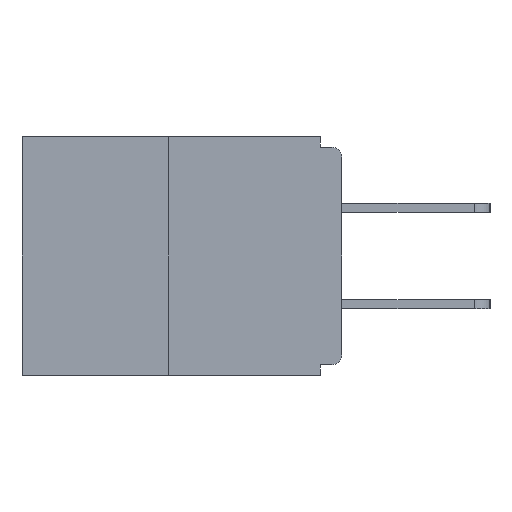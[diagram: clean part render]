
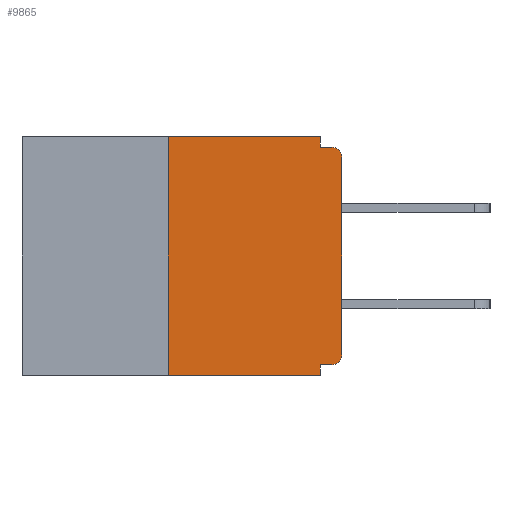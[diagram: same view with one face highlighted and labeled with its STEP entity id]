
A CAD part, left-side view. The second image highlights one B-rep face of the part: STEP entity #9865.
In plain terms, the highlighted planar face has unit normal (-1, 0, 0).
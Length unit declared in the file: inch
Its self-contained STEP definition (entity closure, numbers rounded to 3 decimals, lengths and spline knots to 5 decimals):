
#80 = LINE ( 'NONE', #8680, #6039 ) ;
#93 = DIRECTION ( 'NONE',  ( 1., 0., 0. ) ) ;
#171 = EDGE_CURVE ( 'NONE', #6307, #4086, #8554, .T. ) ;
#205 = CARTESIAN_POINT ( 'NONE',  ( 0., 0.031, -0.328 ) ) ;
#256 = VERTEX_POINT ( 'NONE', #938 ) ;
#393 = CARTESIAN_POINT ( 'NONE',  ( 0., 0.015, -0.015 ) ) ;
#521 = DIRECTION ( 'NONE',  ( 0., -1., 0. ) ) ;
#561 = VERTEX_POINT ( 'NONE', #637 ) ;
#637 = CARTESIAN_POINT ( 'NONE',  ( 0., 0.031, -0.015 ) ) ;
#755 = CARTESIAN_POINT ( 'NONE',  ( 0., 0.25, 0. ) ) ;
#938 = CARTESIAN_POINT ( 'NONE',  ( 0., 0., -0.313 ) ) ;
#1187 = EDGE_CURVE ( 'NONE', #561, #4008, #1650, .T. ) ;
#1219 = EDGE_CURVE ( 'NONE', #5579, #256, #6534, .T. ) ;
#1483 = DIRECTION ( 'NONE',  ( 0., 0., -1. ) ) ;
#1650 = LINE ( 'NONE', #8411, #4233 ) ;
#2197 = VERTEX_POINT ( 'NONE', #205 ) ;
#2252 = CARTESIAN_POINT ( 'NONE',  ( 0., 0.25, 0. ) ) ;
#2537 = CARTESIAN_POINT ( 'NONE',  ( 0., 0.031, 0. ) ) ;
#3429 = CARTESIAN_POINT ( 'NONE',  ( 0., 0.015, -0.313 ) ) ;
#3512 = LINE ( 'NONE', #12268, #11668 ) ;
#3751 = VECTOR ( 'NONE', #4068, 39.37008 ) ;
#4008 = VERTEX_POINT ( 'NONE', #393 ) ;
#4068 = DIRECTION ( 'NONE',  ( 0., 0., 1. ) ) ;
#4086 = VERTEX_POINT ( 'NONE', #2537 ) ;
#4202 = ORIENTED_EDGE ( 'NONE', *, *, #5926, .F. ) ;
#4233 = VECTOR ( 'NONE', #521, 39.37008 ) ;
#4333 = CARTESIAN_POINT ( 'NONE',  ( 0., 0.031, 0. ) ) ;
#4371 = AXIS2_PLACEMENT_3D ( 'NONE', #11123, #12133, #6259 ) ;
#5271 = FACE_OUTER_BOUND ( 'NONE', #10379, .T. ) ;
#5474 = DIRECTION ( 'NONE',  ( 0., 0., -1. ) ) ;
#5579 = VERTEX_POINT ( 'NONE', #8364 ) ;
#5926 = EDGE_CURVE ( 'NONE', #2197, #12095, #3512, .T. ) ;
#6029 = CARTESIAN_POINT ( 'NONE',  ( 0., 0.46, 0. ) ) ;
#6039 = VECTOR ( 'NONE', #9717, 39.37008 ) ;
#6090 = VERTEX_POINT ( 'NONE', #10890 ) ;
#6117 = AXIS2_PLACEMENT_3D ( 'NONE', #3429, #12184, #1483 ) ;
#6259 = DIRECTION ( 'NONE',  ( 0., 0., -1. ) ) ;
#6307 = VERTEX_POINT ( 'NONE', #755 ) ;
#6522 = LINE ( 'NONE', #2252, #3751 ) ;
#6534 = CIRCLE ( 'NONE', #6117, 0.015 ) ;
#6861 = AXIS2_PLACEMENT_3D ( 'NONE', #6029, #93, #10900 ) ;
#6955 = DIRECTION ( 'NONE',  ( 0., -1., 0. ) ) ;
#7190 = CARTESIAN_POINT ( 'NONE',  ( 0., 0., -0.328 ) ) ;
#7238 = CARTESIAN_POINT ( 'NONE',  ( 0., 0.25, -0.343 ) ) ;
#7279 = LINE ( 'NONE', #10842, #11589 ) ;
#7344 = EDGE_CURVE ( 'NONE', #4086, #561, #11327, .T. ) ;
#7654 = ORIENTED_EDGE ( 'NONE', *, *, #7344, .F. ) ;
#7789 = CARTESIAN_POINT ( 'NONE',  ( 0., 0.46, 0. ) ) ;
#7793 = VECTOR ( 'NONE', #12306, 39.37008 ) ;
#7835 = EDGE_CURVE ( 'NONE', #6090, #4008, #9789, .T. ) ;
#7993 = DIRECTION ( 'NONE',  ( 0., 0., 1. ) ) ;
#8178 = DIRECTION ( 'NONE',  ( 0., 1., 0. ) ) ;
#8364 = CARTESIAN_POINT ( 'NONE',  ( 0., 0.015, -0.328 ) ) ;
#8411 = CARTESIAN_POINT ( 'NONE',  ( 0., 0., -0.015 ) ) ;
#8523 = EDGE_CURVE ( 'NONE', #5579, #2197, #11895, .T. ) ;
#8554 = LINE ( 'NONE', #7789, #11791 ) ;
#8680 = CARTESIAN_POINT ( 'NONE',  ( 0., 0.46, -0.343 ) ) ;
#9605 = VECTOR ( 'NONE', #8178, 39.37008 ) ;
#9690 = EDGE_CURVE ( 'NONE', #10013, #12095, #80, .T. ) ;
#9717 = DIRECTION ( 'NONE',  ( 0., -1., 0. ) ) ;
#9789 = CIRCLE ( 'NONE', #4371, 0.015 ) ;
#9865 = ADVANCED_FACE ( 'NONE', ( #5271 ), #9926, .F. ) ;
#9926 = PLANE ( 'NONE',  #6861 ) ;
#10013 = VERTEX_POINT ( 'NONE', #7238 ) ;
#10192 = ORIENTED_EDGE ( 'NONE', *, *, #1219, .T. ) ;
#10379 = EDGE_LOOP ( 'NONE', ( #11484, #11418, #11967, #4202, #12081, #10192, #11290, #12413, #12439, #7654 ) ) ;
#10842 = CARTESIAN_POINT ( 'NONE',  ( 0., 0., 0. ) ) ;
#10890 = CARTESIAN_POINT ( 'NONE',  ( 0., 0., -0.03 ) ) ;
#10900 = DIRECTION ( 'NONE',  ( 0., 0., -1. ) ) ;
#11123 = CARTESIAN_POINT ( 'NONE',  ( 0., 0.015, -0.03 ) ) ;
#11228 = EDGE_CURVE ( 'NONE', #10013, #6307, #6522, .T. ) ;
#11290 = ORIENTED_EDGE ( 'NONE', *, *, #12100, .T. ) ;
#11327 = LINE ( 'NONE', #4333, #7793 ) ;
#11418 = ORIENTED_EDGE ( 'NONE', *, *, #11228, .F. ) ;
#11484 = ORIENTED_EDGE ( 'NONE', *, *, #171, .F. ) ;
#11589 = VECTOR ( 'NONE', #7993, 39.37008 ) ;
#11668 = VECTOR ( 'NONE', #5474, 39.37008 ) ;
#11791 = VECTOR ( 'NONE', #6955, 39.37008 ) ;
#11895 = LINE ( 'NONE', #7190, #9605 ) ;
#11937 = CARTESIAN_POINT ( 'NONE',  ( 0., 0.031, -0.343 ) ) ;
#11967 = ORIENTED_EDGE ( 'NONE', *, *, #9690, .T. ) ;
#12081 = ORIENTED_EDGE ( 'NONE', *, *, #8523, .F. ) ;
#12095 = VERTEX_POINT ( 'NONE', #11937 ) ;
#12100 = EDGE_CURVE ( 'NONE', #256, #6090, #7279, .T. ) ;
#12133 = DIRECTION ( 'NONE',  ( -1., 0., 0. ) ) ;
#12184 = DIRECTION ( 'NONE',  ( -1., 0., 0. ) ) ;
#12268 = CARTESIAN_POINT ( 'NONE',  ( 0., 0.031, -0.343 ) ) ;
#12306 = DIRECTION ( 'NONE',  ( 0., 0., -1. ) ) ;
#12413 = ORIENTED_EDGE ( 'NONE', *, *, #7835, .T. ) ;
#12439 = ORIENTED_EDGE ( 'NONE', *, *, #1187, .F. ) ;
